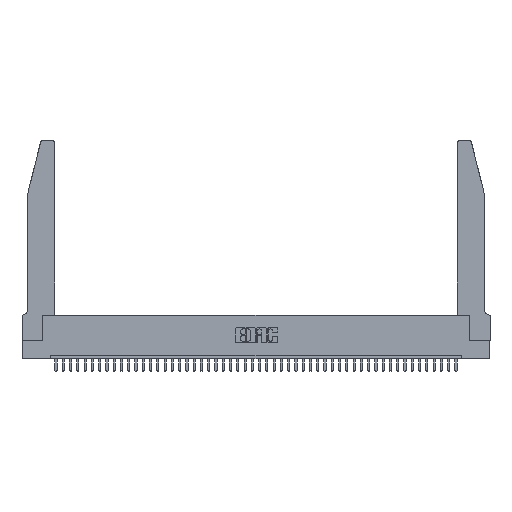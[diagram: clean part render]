
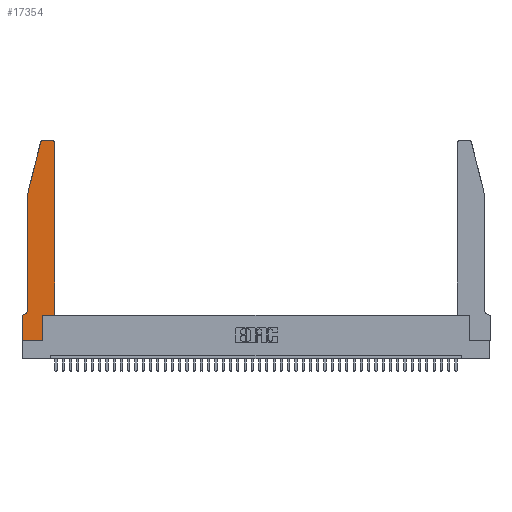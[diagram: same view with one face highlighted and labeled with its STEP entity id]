
A CAD part, top view. The second image highlights one B-rep face of the part: STEP entity #17354.
In plain terms, the highlighted planar face has unit normal (0, 0, 1).
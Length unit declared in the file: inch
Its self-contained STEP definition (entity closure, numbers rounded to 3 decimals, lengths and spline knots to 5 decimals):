
#297 = CARTESIAN_POINT ( 'NONE',  ( 0., 0., 0.37 ) ) ;
#829 = CARTESIAN_POINT ( 'NONE',  ( 0., 0., 0.37 ) ) ;
#2806 = EDGE_CURVE ( 'NONE', #11590, #20776, #13260, .T. ) ;
#3514 = LINE ( 'NONE', #33676, #15563 ) ;
#4814 = CARTESIAN_POINT ( 'NONE',  ( 0.0055, 0.35, 0.37 ) ) ;
#5041 = VERTEX_POINT ( 'NONE', #6527 ) ;
#5295 = DIRECTION ( 'NONE',  ( 0., -1., 0. ) ) ;
#6059 = AXIS2_PLACEMENT_3D ( 'NONE', #30912, #27105, #23425 ) ;
#6527 = CARTESIAN_POINT ( 'NONE',  ( 0.0755, 2., 0.37 ) ) ;
#7048 = VECTOR ( 'NONE', #27621, 39.37008 ) ;
#7082 = EDGE_CURVE ( 'NONE', #16627, #5041, #12533, .T. ) ;
#7386 = CARTESIAN_POINT ( 'NONE',  ( 0., 0.35, 0.37 ) ) ;
#7700 = EDGE_CURVE ( 'NONE', #34144, #11590, #38642, .T. ) ;
#7778 = VERTEX_POINT ( 'NONE', #44641 ) ;
#7941 = CARTESIAN_POINT ( 'NONE',  ( 0.284, 2.75, 0.37 ) ) ;
#8201 = CARTESIAN_POINT ( 'NONE',  ( 0.4205, 2.75, 0.37 ) ) ;
#8626 = DIRECTION ( 'NONE',  ( 0., 0., 1. ) ) ;
#8726 = ORIENTED_EDGE ( 'NONE', *, *, #2806, .T. ) ;
#8870 = VERTEX_POINT ( 'NONE', #7941 ) ;
#10557 = DIRECTION ( 'NONE',  ( 0., 0., 1. ) ) ;
#10852 = VECTOR ( 'NONE', #28696, 39.37008 ) ;
#11020 = CARTESIAN_POINT ( 'NONE',  ( 0.284, 2.72, 0.37 ) ) ;
#11258 = VERTEX_POINT ( 'NONE', #38142 ) ;
#11590 = VERTEX_POINT ( 'NONE', #42153 ) ;
#12533 = LINE ( 'NONE', #25318, #26773 ) ;
#12543 = EDGE_CURVE ( 'NONE', #11258, #35841, #26179, .T. ) ;
#12746 = DIRECTION ( 'NONE',  ( 0., -1., 0. ) ) ;
#13260 = LINE ( 'NONE', #35869, #21509 ) ;
#13299 = VERTEX_POINT ( 'NONE', #4814 ) ;
#14103 = VECTOR ( 'NONE', #21271, 39.37008 ) ;
#14124 = VECTOR ( 'NONE', #27320, 39.37008 ) ;
#14130 = PLANE ( 'NONE',  #27925 ) ;
#14405 = DIRECTION ( 'NONE',  ( -1., 0., 0. ) ) ;
#14578 = DIRECTION ( 'NONE',  ( -0.239, -0.971, 0. ) ) ;
#15563 = VECTOR ( 'NONE', #12746, 39.37008 ) ;
#15855 = CARTESIAN_POINT ( 'NONE',  ( 0., 0., 0.37 ) ) ;
#16172 = ORIENTED_EDGE ( 'NONE', *, *, #19664, .T. ) ;
#16519 = CARTESIAN_POINT ( 'NONE',  ( 0.2865, 0., 0.37 ) ) ;
#16627 = VERTEX_POINT ( 'NONE', #42944 ) ;
#17354 = ADVANCED_FACE ( 'NONE', ( #40469 ), #14130, .T. ) ;
#17654 = VERTEX_POINT ( 'NONE', #8201 ) ;
#18954 = EDGE_CURVE ( 'NONE', #35841, #34144, #33817, .T. ) ;
#19664 = EDGE_CURVE ( 'NONE', #5041, #28092, #3514, .T. ) ;
#20734 = CIRCLE ( 'NONE', #24681, 0.03 ) ;
#20776 = VERTEX_POINT ( 'NONE', #27354 ) ;
#20783 = ORIENTED_EDGE ( 'NONE', *, *, #18954, .T. ) ;
#20813 = LINE ( 'NONE', #41584, #7048 ) ;
#20819 = EDGE_LOOP ( 'NONE', ( #38622, #29969, #28416, #16172, #32444, #23534, #36040, #20783, #33771, #8726, #35967, #28882 ) ) ;
#21271 = DIRECTION ( 'NONE',  ( 0., 1., 0. ) ) ;
#21509 = VECTOR ( 'NONE', #22020, 39.37008 ) ;
#22020 = DIRECTION ( 'NONE',  ( 1., 0., 0. ) ) ;
#23425 = DIRECTION ( 'NONE',  ( -1., 0., 0. ) ) ;
#23468 = EDGE_CURVE ( 'NONE', #7778, #17654, #31559, .T. ) ;
#23534 = ORIENTED_EDGE ( 'NONE', *, *, #30617, .T. ) ;
#24025 = VECTOR ( 'NONE', #5295, 39.37008 ) ;
#24344 = VECTOR ( 'NONE', #14405, 39.37008 ) ;
#24681 = AXIS2_PLACEMENT_3D ( 'NONE', #11020, #10557, #35433 ) ;
#24729 = DIRECTION ( 'NONE',  ( 1., 0., 0. ) ) ;
#25318 = CARTESIAN_POINT ( 'NONE',  ( 0.0755, 2., 0.37 ) ) ;
#26103 = DIRECTION ( 'NONE',  ( 1., 0., 0. ) ) ;
#26179 = LINE ( 'NONE', #15855, #24025 ) ;
#26216 = LINE ( 'NONE', #34462, #14124 ) ;
#26773 = VECTOR ( 'NONE', #14578, 39.37008 ) ;
#27105 = DIRECTION ( 'NONE',  ( 0., 0., -1. ) ) ;
#27320 = DIRECTION ( 'NONE',  ( -1., 0., 0. ) ) ;
#27354 = CARTESIAN_POINT ( 'NONE',  ( 0.4505, 0.35, 0.37 ) ) ;
#27621 = DIRECTION ( 'NONE',  ( 0., 1., 0. ) ) ;
#27925 = AXIS2_PLACEMENT_3D ( 'NONE', #7386, #34905, #24729 ) ;
#28092 = VERTEX_POINT ( 'NONE', #43472 ) ;
#28314 = CARTESIAN_POINT ( 'NONE',  ( 0.2605, 2.75, 0.37 ) ) ;
#28416 = ORIENTED_EDGE ( 'NONE', *, *, #7082, .T. ) ;
#28696 = DIRECTION ( 'NONE',  ( 1., 0., 0. ) ) ;
#28882 = ORIENTED_EDGE ( 'NONE', *, *, #23468, .T. ) ;
#29969 = ORIENTED_EDGE ( 'NONE', *, *, #35268, .T. ) ;
#30183 = EDGE_CURVE ( 'NONE', #20776, #7778, #20813, .T. ) ;
#30617 = EDGE_CURVE ( 'NONE', #13299, #11258, #26216, .T. ) ;
#30912 = CARTESIAN_POINT ( 'NONE',  ( 0.0055, 0.42, 0.37 ) ) ;
#31368 = CARTESIAN_POINT ( 'NONE',  ( 0.2865, 0.35, 0.37 ) ) ;
#31559 = CIRCLE ( 'NONE', #42098, 0.03 ) ;
#32444 = ORIENTED_EDGE ( 'NONE', *, *, #42456, .T. ) ;
#32926 = EDGE_CURVE ( 'NONE', #17654, #8870, #40617, .T. ) ;
#33676 = CARTESIAN_POINT ( 'NONE',  ( 0.0755, 2., 0.37 ) ) ;
#33771 = ORIENTED_EDGE ( 'NONE', *, *, #7700, .T. ) ;
#33817 = LINE ( 'NONE', #297, #10852 ) ;
#34144 = VERTEX_POINT ( 'NONE', #16519 ) ;
#34462 = CARTESIAN_POINT ( 'NONE',  ( 0.0755, 0.35, 0.37 ) ) ;
#34905 = DIRECTION ( 'NONE',  ( 0., 0., 1. ) ) ;
#35268 = EDGE_CURVE ( 'NONE', #8870, #16627, #20734, .T. ) ;
#35433 = DIRECTION ( 'NONE',  ( 1., 0., 0. ) ) ;
#35841 = VERTEX_POINT ( 'NONE', #829 ) ;
#35869 = CARTESIAN_POINT ( 'NONE',  ( 0.4505, 0.35, 0.37 ) ) ;
#35967 = ORIENTED_EDGE ( 'NONE', *, *, #30183, .T. ) ;
#36040 = ORIENTED_EDGE ( 'NONE', *, *, #12543, .T. ) ;
#36468 = CARTESIAN_POINT ( 'NONE',  ( 0.4205, 2.72, 0.37 ) ) ;
#38142 = CARTESIAN_POINT ( 'NONE',  ( 0., 0.35, 0.37 ) ) ;
#38622 = ORIENTED_EDGE ( 'NONE', *, *, #32926, .T. ) ;
#38642 = LINE ( 'NONE', #31368, #14103 ) ;
#40469 = FACE_OUTER_BOUND ( 'NONE', #20819, .T. ) ;
#40617 = LINE ( 'NONE', #28314, #24344 ) ;
#41584 = CARTESIAN_POINT ( 'NONE',  ( 0.4505, 0.35, 0.37 ) ) ;
#42098 = AXIS2_PLACEMENT_3D ( 'NONE', #36468, #8626, #26103 ) ;
#42153 = CARTESIAN_POINT ( 'NONE',  ( 0.2865, 0.35, 0.37 ) ) ;
#42456 = EDGE_CURVE ( 'NONE', #28092, #13299, #42970, .T. ) ;
#42944 = CARTESIAN_POINT ( 'NONE',  ( 0.25487, 2.72718, 0.37 ) ) ;
#42970 = CIRCLE ( 'NONE', #6059, 0.07 ) ;
#43472 = CARTESIAN_POINT ( 'NONE',  ( 0.0755, 0.42, 0.37 ) ) ;
#44641 = CARTESIAN_POINT ( 'NONE',  ( 0.4505, 2.72, 0.37 ) ) ;
